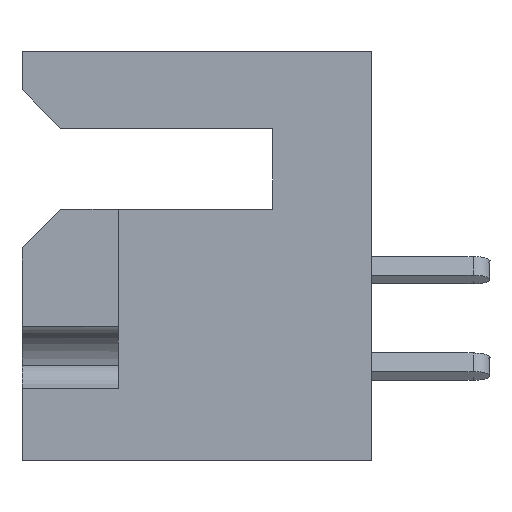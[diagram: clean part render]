
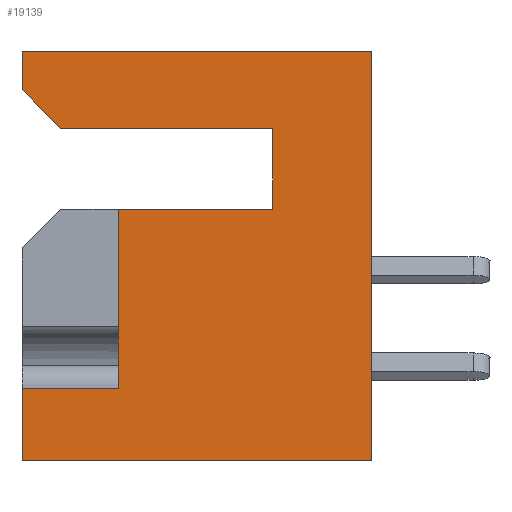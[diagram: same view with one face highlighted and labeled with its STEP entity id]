
A CAD part, left-side view. The second image highlights one B-rep face of the part: STEP entity #19139.
In plain terms, the highlighted planar face has unit normal (-1, 0, 0).
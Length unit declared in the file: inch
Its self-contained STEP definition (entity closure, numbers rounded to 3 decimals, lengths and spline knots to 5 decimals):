
#110 = ORIENTED_EDGE ( 'NONE', *, *, #15637, .F. ) ;
#137 = CARTESIAN_POINT ( 'NONE',  ( 0., 0.128, -0.205 ) ) ;
#222 = PLANE ( 'NONE',  #19488 ) ;
#1069 = VERTEX_POINT ( 'NONE', #21569 ) ;
#1099 = CARTESIAN_POINT ( 'NONE',  ( 0., 0., 0. ) ) ;
#1731 = ORIENTED_EDGE ( 'NONE', *, *, #14404, .F. ) ;
#1865 = VERTEX_POINT ( 'NONE', #17096 ) ;
#2281 = CARTESIAN_POINT ( 'NONE',  ( 0., 0.453, -0.05 ) ) ;
#2297 = DIRECTION ( 'NONE',  ( 0., -1., 0. ) ) ;
#2408 = DIRECTION ( 'NONE',  ( 0., 0., -1. ) ) ;
#3046 = VERTEX_POINT ( 'NONE', #137 ) ;
#3318 = VERTEX_POINT ( 'NONE', #10823 ) ;
#3351 = ORIENTED_EDGE ( 'NONE', *, *, #18355, .F. ) ;
#3846 = ORIENTED_EDGE ( 'NONE', *, *, #14783, .F. ) ;
#3880 = EDGE_CURVE ( 'NONE', #21070, #25872, #16419, .T. ) ;
#4190 = CARTESIAN_POINT ( 'NONE',  ( 0., 0.453, 0. ) ) ;
#4372 = LINE ( 'NONE', #14884, #16555 ) ;
#4376 = ORIENTED_EDGE ( 'NONE', *, *, #17013, .T. ) ;
#4452 = DIRECTION ( 'NONE',  ( 1., 0., 0. ) ) ;
#4998 = VECTOR ( 'NONE', #25999, 39.37008 ) ;
#5058 = CARTESIAN_POINT ( 'NONE',  ( 0., 0., 0. ) ) ;
#5321 = CARTESIAN_POINT ( 'NONE',  ( 0., 0.453, 0. ) ) ;
#5335 = LINE ( 'NONE', #4190, #20522 ) ;
#5362 = DIRECTION ( 'NONE',  ( 0., 1., 0. ) ) ;
#5889 = VERTEX_POINT ( 'NONE', #5321 ) ;
#6065 = VECTOR ( 'NONE', #26171, 39.37008 ) ;
#6804 = EDGE_CURVE ( 'NONE', #1865, #19289, #7072, .T. ) ;
#7072 = LINE ( 'NONE', #23534, #26487 ) ;
#7192 = LINE ( 'NONE', #19160, #21706 ) ;
#8177 = DIRECTION ( 'NONE',  ( 0., 0., 1. ) ) ;
#8184 = VECTOR ( 'NONE', #19957, 39.37008 ) ;
#8790 = EDGE_CURVE ( 'NONE', #1069, #17740, #23091, .T. ) ;
#8928 = DIRECTION ( 'NONE',  ( 0., 1., 0. ) ) ;
#9261 = CARTESIAN_POINT ( 'NONE',  ( 0., 0.128, -0.1 ) ) ;
#9781 = ORIENTED_EDGE ( 'NONE', *, *, #6804, .F. ) ;
#10147 = VECTOR ( 'NONE', #2297, 39.37008 ) ;
#10252 = ORIENTED_EDGE ( 'NONE', *, *, #3880, .T. ) ;
#10823 = CARTESIAN_POINT ( 'NONE',  ( 0., 0.453, -0.437 ) ) ;
#11563 = LINE ( 'NONE', #22304, #19187 ) ;
#13001 = DIRECTION ( 'NONE',  ( 0., 0., 1. ) ) ;
#13704 = DIRECTION ( 'NONE',  ( 0., -1., 0. ) ) ;
#13717 = CARTESIAN_POINT ( 'NONE',  ( 0., 0.128, -0.1 ) ) ;
#13989 = VERTEX_POINT ( 'NONE', #1099 ) ;
#14404 = EDGE_CURVE ( 'NONE', #19819, #5889, #4372, .T. ) ;
#14644 = EDGE_CURVE ( 'NONE', #1865, #3318, #17861, .T. ) ;
#14783 = EDGE_CURVE ( 'NONE', #5889, #13989, #11563, .T. ) ;
#14798 = DIRECTION ( 'NONE',  ( 0., 0., 1. ) ) ;
#14884 = CARTESIAN_POINT ( 'NONE',  ( 0., 0.453, 0. ) ) ;
#15387 = CARTESIAN_POINT ( 'NONE',  ( 0., 0.328, -0.205 ) ) ;
#15637 = EDGE_CURVE ( 'NONE', #21070, #3318, #5335, .T. ) ;
#15871 = ORIENTED_EDGE ( 'NONE', *, *, #20854, .T. ) ;
#16419 = LINE ( 'NONE', #19451, #10147 ) ;
#16555 = VECTOR ( 'NONE', #14798, 39.37008 ) ;
#16805 = CARTESIAN_POINT ( 'NONE',  ( 0., 0.453, 0. ) ) ;
#17013 = EDGE_CURVE ( 'NONE', #3046, #19289, #21470, .T. ) ;
#17096 = CARTESIAN_POINT ( 'NONE',  ( 0., 0.328, -0.437 ) ) ;
#17520 = CARTESIAN_POINT ( 'NONE',  ( 0., 0.403, -0.1 ) ) ;
#17702 = ORIENTED_EDGE ( 'NONE', *, *, #18058, .T. ) ;
#17714 = FACE_OUTER_BOUND ( 'NONE', #25343, .T. ) ;
#17740 = VERTEX_POINT ( 'NONE', #17520 ) ;
#17861 = LINE ( 'NONE', #23892, #4998 ) ;
#18058 = EDGE_CURVE ( 'NONE', #19819, #17740, #7192, .T. ) ;
#18355 = EDGE_CURVE ( 'NONE', #3046, #1069, #26317, .T. ) ;
#18769 = ORIENTED_EDGE ( 'NONE', *, *, #14644, .T. ) ;
#18801 = CARTESIAN_POINT ( 'NONE',  ( 0., 0.453, -0.531 ) ) ;
#19139 = ADVANCED_FACE ( 'NONE', ( #17714 ), #222, .F. ) ;
#19160 = CARTESIAN_POINT ( 'NONE',  ( 0., 0.403, -0.1 ) ) ;
#19187 = VECTOR ( 'NONE', #13704, 39.37008 ) ;
#19209 = ORIENTED_EDGE ( 'NONE', *, *, #8790, .F. ) ;
#19289 = VERTEX_POINT ( 'NONE', #15387 ) ;
#19451 = CARTESIAN_POINT ( 'NONE',  ( 0., 0.453, -0.531 ) ) ;
#19488 = AXIS2_PLACEMENT_3D ( 'NONE', #16805, #4452, #2408 ) ;
#19819 = VERTEX_POINT ( 'NONE', #2281 ) ;
#19957 = DIRECTION ( 'NONE',  ( 0., 0., 1. ) ) ;
#20522 = VECTOR ( 'NONE', #8177, 39.37008 ) ;
#20809 = VECTOR ( 'NONE', #8928, 39.37008 ) ;
#20854 = EDGE_CURVE ( 'NONE', #25872, #13989, #26490, .T. ) ;
#21070 = VERTEX_POINT ( 'NONE', #18801 ) ;
#21470 = LINE ( 'NONE', #25701, #20809 ) ;
#21569 = CARTESIAN_POINT ( 'NONE',  ( 0., 0.128, -0.1 ) ) ;
#21706 = VECTOR ( 'NONE', #27254, 39.37008 ) ;
#22304 = CARTESIAN_POINT ( 'NONE',  ( 0., 0.453, 0. ) ) ;
#23091 = LINE ( 'NONE', #13717, #25724 ) ;
#23534 = CARTESIAN_POINT ( 'NONE',  ( 0., 0.328, -0.205 ) ) ;
#23892 = CARTESIAN_POINT ( 'NONE',  ( 0., 0.328, -0.437 ) ) ;
#25343 = EDGE_LOOP ( 'NONE', ( #18769, #110, #10252, #15871, #3846, #1731, #17702, #19209, #3351, #4376, #9781 ) ) ;
#25701 = CARTESIAN_POINT ( 'NONE',  ( 0., 0.128, -0.205 ) ) ;
#25724 = VECTOR ( 'NONE', #5362, 39.37008 ) ;
#25872 = VERTEX_POINT ( 'NONE', #25887 ) ;
#25887 = CARTESIAN_POINT ( 'NONE',  ( 0., 0., -0.531 ) ) ;
#25999 = DIRECTION ( 'NONE',  ( 0., 1., 0. ) ) ;
#26171 = DIRECTION ( 'NONE',  ( 0., 0., 1. ) ) ;
#26317 = LINE ( 'NONE', #9261, #8184 ) ;
#26487 = VECTOR ( 'NONE', #13001, 39.37008 ) ;
#26490 = LINE ( 'NONE', #5058, #6065 ) ;
#27254 = DIRECTION ( 'NONE',  ( 0., -0.707, -0.707 ) ) ;
